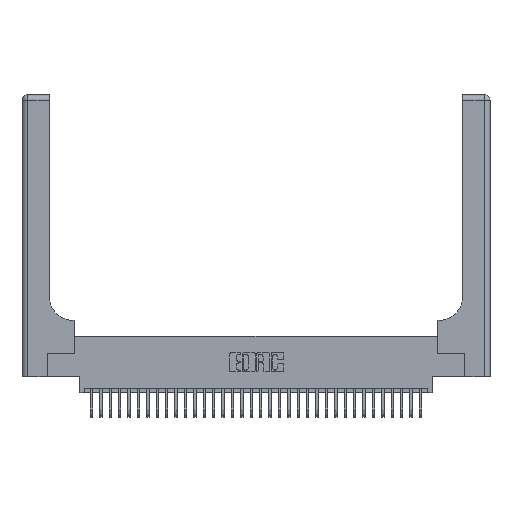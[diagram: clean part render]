
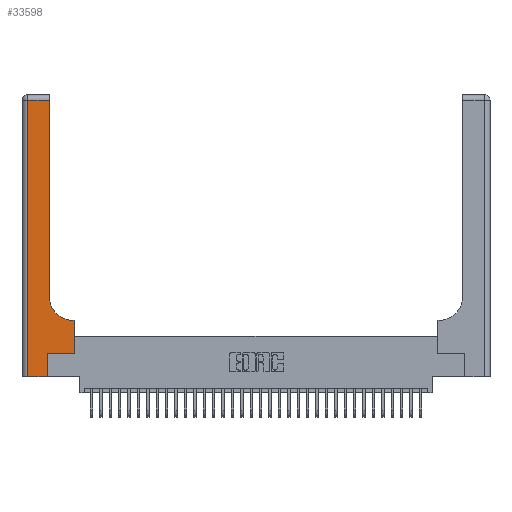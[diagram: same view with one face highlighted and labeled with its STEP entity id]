
A CAD part, top view. The second image highlights one B-rep face of the part: STEP entity #33598.
In plain terms, the highlighted planar face has unit normal (0, 0, 1).
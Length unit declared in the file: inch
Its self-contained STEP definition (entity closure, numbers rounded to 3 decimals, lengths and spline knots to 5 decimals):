
#510 = LINE ( 'NONE', #11065, #30192 ) ;
#961 = LINE ( 'NONE', #4111, #16682 ) ;
#2382 = VECTOR ( 'NONE', #35291, 39.37008 ) ;
#2730 = EDGE_CURVE ( 'NONE', #32063, #16110, #510, .T. ) ;
#3904 = VERTEX_POINT ( 'NONE', #15862 ) ;
#4023 = ORIENTED_EDGE ( 'NONE', *, *, #18738, .T. ) ;
#4111 = CARTESIAN_POINT ( 'NONE',  ( 0.2915, 3., 0.37 ) ) ;
#4522 = EDGE_CURVE ( 'NONE', #17864, #13335, #21970, .T. ) ;
#4536 = CARTESIAN_POINT ( 'NONE',  ( 0., 2.94, 0.37 ) ) ;
#5711 = VECTOR ( 'NONE', #10781, 39.37008 ) ;
#5765 = EDGE_CURVE ( 'NONE', #16110, #30281, #27995, .T. ) ;
#6861 = CARTESIAN_POINT ( 'NONE',  ( 0.5585, 0.25, 0.37 ) ) ;
#7775 = EDGE_LOOP ( 'NONE', ( #17834, #26952, #17614, #34339, #4023, #13346, #30299, #28522, #33390 ) ) ;
#7956 = CARTESIAN_POINT ( 'NONE',  ( 0., 0., 0.37 ) ) ;
#10028 = DIRECTION ( 'NONE',  ( 0., 0., -1. ) ) ;
#10498 = VECTOR ( 'NONE', #30806, 39.37008 ) ;
#10781 = DIRECTION ( 'NONE',  ( 1., 0., 0. ) ) ;
#10894 = CARTESIAN_POINT ( 'NONE',  ( 0.5585, 0.6, 0.37 ) ) ;
#11065 = CARTESIAN_POINT ( 'NONE',  ( 0.2915, 0.6, 0.37 ) ) ;
#11512 = EDGE_CURVE ( 'NONE', #29939, #3904, #23781, .T. ) ;
#12119 = DIRECTION ( 'NONE',  ( -1., 0., 0. ) ) ;
#12645 = AXIS2_PLACEMENT_3D ( 'NONE', #28694, #28819, #12119 ) ;
#12877 = CARTESIAN_POINT ( 'NONE',  ( 0.269, 0.25, 0.37 ) ) ;
#13335 = VERTEX_POINT ( 'NONE', #6861 ) ;
#13346 = ORIENTED_EDGE ( 'NONE', *, *, #4522, .T. ) ;
#14128 = EDGE_CURVE ( 'NONE', #31521, #33821, #35322, .T. ) ;
#14538 = DIRECTION ( 'NONE',  ( 0., -1., 0. ) ) ;
#15460 = EDGE_CURVE ( 'NONE', #13335, #32063, #30976, .T. ) ;
#15862 = CARTESIAN_POINT ( 'NONE',  ( 0.06, 2.94, 0.37 ) ) ;
#16110 = VERTEX_POINT ( 'NONE', #25621 ) ;
#16682 = VECTOR ( 'NONE', #23612, 39.37008 ) ;
#16833 = EDGE_CURVE ( 'NONE', #3904, #31521, #32597, .T. ) ;
#16878 = CARTESIAN_POINT ( 'NONE',  ( 0.269, 0.25, 0.37 ) ) ;
#17269 = VECTOR ( 'NONE', #18443, 39.37008 ) ;
#17614 = ORIENTED_EDGE ( 'NONE', *, *, #16833, .T. ) ;
#17834 = ORIENTED_EDGE ( 'NONE', *, *, #35202, .T. ) ;
#17864 = VERTEX_POINT ( 'NONE', #16878 ) ;
#17977 = CARTESIAN_POINT ( 'NONE',  ( 0.2915, 2.94, 0.37 ) ) ;
#18443 = DIRECTION ( 'NONE',  ( -1., 0., 0. ) ) ;
#18738 = EDGE_CURVE ( 'NONE', #33821, #17864, #23744, .T. ) ;
#21970 = LINE ( 'NONE', #12877, #29383 ) ;
#23242 = FACE_OUTER_BOUND ( 'NONE', #7775, .T. ) ;
#23437 = VECTOR ( 'NONE', #14538, 39.37008 ) ;
#23612 = DIRECTION ( 'NONE',  ( 0., 1., 0. ) ) ;
#23744 = LINE ( 'NONE', #26929, #2382 ) ;
#23781 = LINE ( 'NONE', #4536, #17269 ) ;
#25621 = CARTESIAN_POINT ( 'NONE',  ( 0.5415, 0.6, 0.37 ) ) ;
#26013 = PLANE ( 'NONE',  #12645 ) ;
#26718 = CARTESIAN_POINT ( 'NONE',  ( 0.5415, 0.85, 0.37 ) ) ;
#26929 = CARTESIAN_POINT ( 'NONE',  ( 0.269, 0., 0.37 ) ) ;
#26952 = ORIENTED_EDGE ( 'NONE', *, *, #11512, .T. ) ;
#26968 = CARTESIAN_POINT ( 'NONE',  ( 0.269, 0., 0.37 ) ) ;
#27450 = AXIS2_PLACEMENT_3D ( 'NONE', #26718, #10028, #29505 ) ;
#27995 = CIRCLE ( 'NONE', #27450, 0.25 ) ;
#27996 = CARTESIAN_POINT ( 'NONE',  ( 0.5585, 0.25, 0.37 ) ) ;
#28522 = ORIENTED_EDGE ( 'NONE', *, *, #2730, .T. ) ;
#28694 = CARTESIAN_POINT ( 'NONE',  ( 0., 3., 0.37 ) ) ;
#28819 = DIRECTION ( 'NONE',  ( 0., 0., -1. ) ) ;
#29383 = VECTOR ( 'NONE', #32354, 39.37008 ) ;
#29505 = DIRECTION ( 'NONE',  ( 1., 0., 0. ) ) ;
#29939 = VERTEX_POINT ( 'NONE', #17977 ) ;
#30192 = VECTOR ( 'NONE', #30554, 39.37008 ) ;
#30281 = VERTEX_POINT ( 'NONE', #35372 ) ;
#30299 = ORIENTED_EDGE ( 'NONE', *, *, #15460, .T. ) ;
#30554 = DIRECTION ( 'NONE',  ( -1., 0., 0. ) ) ;
#30806 = DIRECTION ( 'NONE',  ( 0., 1., 0. ) ) ;
#30976 = LINE ( 'NONE', #27996, #10498 ) ;
#31521 = VERTEX_POINT ( 'NONE', #33548 ) ;
#32063 = VERTEX_POINT ( 'NONE', #10894 ) ;
#32354 = DIRECTION ( 'NONE',  ( 1., 0., 0. ) ) ;
#32597 = LINE ( 'NONE', #33976, #23437 ) ;
#33390 = ORIENTED_EDGE ( 'NONE', *, *, #5765, .T. ) ;
#33548 = CARTESIAN_POINT ( 'NONE',  ( 0.06, 0., 0.37 ) ) ;
#33598 = ADVANCED_FACE ( 'NONE', ( #23242 ), #26013, .F. ) ;
#33821 = VERTEX_POINT ( 'NONE', #26968 ) ;
#33976 = CARTESIAN_POINT ( 'NONE',  ( 0.06, 3., 0.37 ) ) ;
#34339 = ORIENTED_EDGE ( 'NONE', *, *, #14128, .T. ) ;
#35202 = EDGE_CURVE ( 'NONE', #30281, #29939, #961, .T. ) ;
#35291 = DIRECTION ( 'NONE',  ( 0., 1., 0. ) ) ;
#35322 = LINE ( 'NONE', #7956, #5711 ) ;
#35372 = CARTESIAN_POINT ( 'NONE',  ( 0.2915, 0.85, 0.37 ) ) ;
